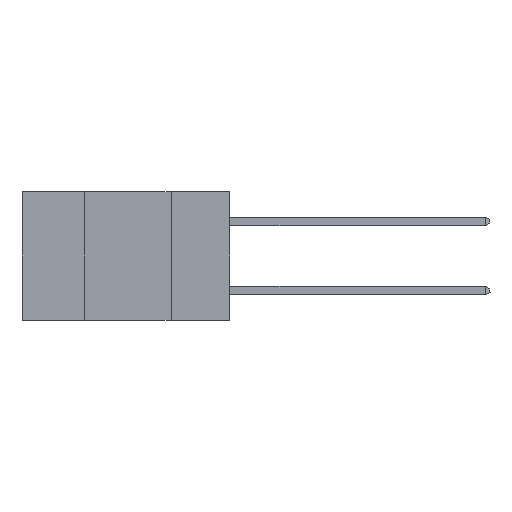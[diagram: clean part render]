
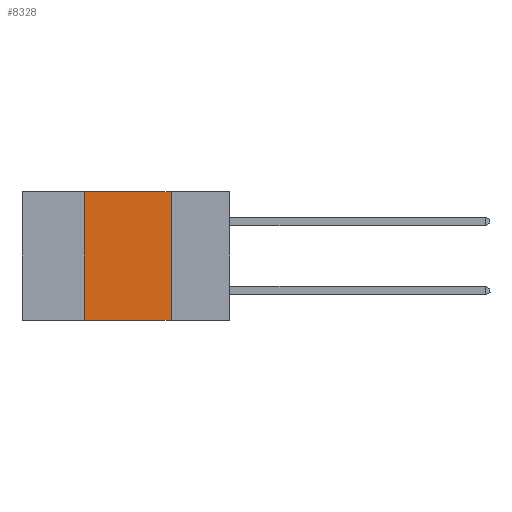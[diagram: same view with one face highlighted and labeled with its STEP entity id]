
A CAD part, left-side view. The second image highlights one B-rep face of the part: STEP entity #8328.
In plain terms, the highlighted planar face has unit normal (-1, 0, 0).
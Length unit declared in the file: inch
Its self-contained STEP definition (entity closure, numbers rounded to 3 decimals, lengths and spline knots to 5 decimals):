
#25 = VECTOR ( 'NONE', #5046, 39.37008 ) ;
#218 = DIRECTION ( 'NONE',  ( 0., 0., 1. ) ) ;
#494 = CARTESIAN_POINT ( 'NONE',  ( 0., 0.6, 0. ) ) ;
#870 = VERTEX_POINT ( 'NONE', #6539 ) ;
#947 = CARTESIAN_POINT ( 'NONE',  ( 0., 0.42, 0. ) ) ;
#1298 = DIRECTION ( 'NONE',  ( 0., 0., -1. ) ) ;
#1325 = DIRECTION ( 'NONE',  ( 0., -1., 0. ) ) ;
#2252 = EDGE_CURVE ( 'NONE', #4037, #870, #9722, .T. ) ;
#2342 = CARTESIAN_POINT ( 'NONE',  ( 0., 0.17, 0. ) ) ;
#2723 = CARTESIAN_POINT ( 'NONE',  ( 0., 0.17, 0. ) ) ;
#2762 = ORIENTED_EDGE ( 'NONE', *, *, #8362, .F. ) ;
#2827 = ORIENTED_EDGE ( 'NONE', *, *, #2947, .F. ) ;
#2947 = EDGE_CURVE ( 'NONE', #8878, #870, #4253, .T. ) ;
#3313 = CARTESIAN_POINT ( 'NONE',  ( 0., 0.6, 0. ) ) ;
#3380 = PLANE ( 'NONE',  #9528 ) ;
#4037 = VERTEX_POINT ( 'NONE', #4567 ) ;
#4162 = DIRECTION ( 'NONE',  ( 0., 0., -1. ) ) ;
#4253 = LINE ( 'NONE', #2723, #10362 ) ;
#4567 = CARTESIAN_POINT ( 'NONE',  ( 0., 0.42, -0.37 ) ) ;
#4650 = CARTESIAN_POINT ( 'NONE',  ( 0., 0.6, -0.37 ) ) ;
#4728 = VECTOR ( 'NONE', #1325, 39.37008 ) ;
#4993 = DIRECTION ( 'NONE',  ( 1., 0., 0. ) ) ;
#5046 = DIRECTION ( 'NONE',  ( 0., -1., 0. ) ) ;
#5186 = VERTEX_POINT ( 'NONE', #9550 ) ;
#5798 = FACE_OUTER_BOUND ( 'NONE', #7840, .T. ) ;
#6220 = ORIENTED_EDGE ( 'NONE', *, *, #10227, .F. ) ;
#6539 = CARTESIAN_POINT ( 'NONE',  ( 0., 0.17, -0.37 ) ) ;
#7380 = LINE ( 'NONE', #494, #4728 ) ;
#7840 = EDGE_LOOP ( 'NONE', ( #2827, #6220, #2762, #10007 ) ) ;
#8328 = ADVANCED_FACE ( 'NONE', ( #5798 ), #3380, .F. ) ;
#8362 = EDGE_CURVE ( 'NONE', #4037, #5186, #8712, .T. ) ;
#8712 = LINE ( 'NONE', #947, #9225 ) ;
#8878 = VERTEX_POINT ( 'NONE', #2342 ) ;
#9225 = VECTOR ( 'NONE', #218, 39.37008 ) ;
#9528 = AXIS2_PLACEMENT_3D ( 'NONE', #3313, #4993, #4162 ) ;
#9550 = CARTESIAN_POINT ( 'NONE',  ( 0., 0.42, 0. ) ) ;
#9722 = LINE ( 'NONE', #4650, #25 ) ;
#10007 = ORIENTED_EDGE ( 'NONE', *, *, #2252, .T. ) ;
#10227 = EDGE_CURVE ( 'NONE', #5186, #8878, #7380, .T. ) ;
#10362 = VECTOR ( 'NONE', #1298, 39.37008 ) ;
